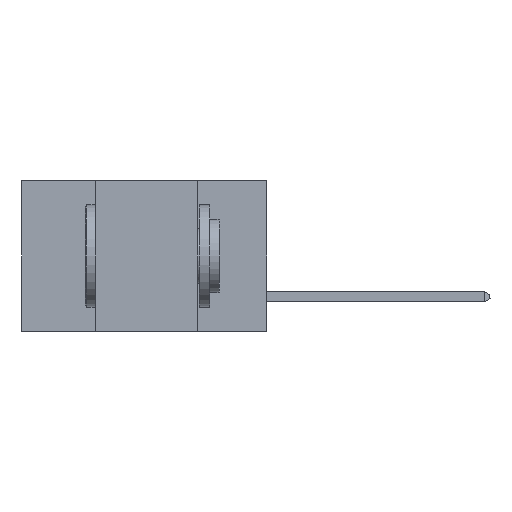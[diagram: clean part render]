
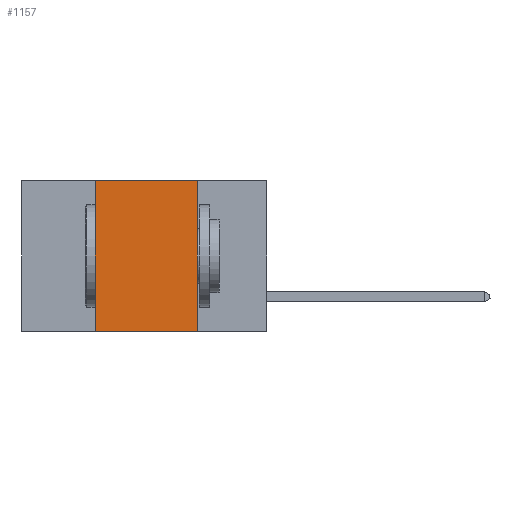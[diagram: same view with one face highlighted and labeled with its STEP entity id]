
A CAD part, left-side view. The second image highlights one B-rep face of the part: STEP entity #1157.
In plain terms, the highlighted planar face has unit normal (-1, 0, 0).
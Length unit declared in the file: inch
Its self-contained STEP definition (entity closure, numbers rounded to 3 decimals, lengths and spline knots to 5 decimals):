
#490 = ORIENTED_EDGE ( 'NONE', *, *, #20803, .F. ) ;
#624 = LINE ( 'NONE', #4602, #13449 ) ;
#963 = CARTESIAN_POINT ( 'NONE',  ( 0., 0.42, -0.37 ) ) ;
#1157 = ADVANCED_FACE ( 'NONE', ( #11332 ), #4888, .F. ) ;
#2945 = DIRECTION ( 'NONE',  ( 0., 0., 1. ) ) ;
#3739 = DIRECTION ( 'NONE',  ( 0., 0., -1. ) ) ;
#4158 = VERTEX_POINT ( 'NONE', #963 ) ;
#4268 = DIRECTION ( 'NONE',  ( 1., 0., 0. ) ) ;
#4602 = CARTESIAN_POINT ( 'NONE',  ( 0., 0.42, 0. ) ) ;
#4737 = CARTESIAN_POINT ( 'NONE',  ( 0., 0.6, 0. ) ) ;
#4888 = PLANE ( 'NONE',  #20525 ) ;
#5513 = VERTEX_POINT ( 'NONE', #19071 ) ;
#6127 = LINE ( 'NONE', #12574, #18599 ) ;
#7442 = EDGE_CURVE ( 'NONE', #8798, #15457, #12345, .T. ) ;
#8257 = DIRECTION ( 'NONE',  ( 0., -1., 0. ) ) ;
#8798 = VERTEX_POINT ( 'NONE', #10194 ) ;
#8953 = VECTOR ( 'NONE', #15605, 39.37008 ) ;
#10194 = CARTESIAN_POINT ( 'NONE',  ( 0., 0.17, 0. ) ) ;
#11332 = FACE_OUTER_BOUND ( 'NONE', #11573, .T. ) ;
#11573 = EDGE_LOOP ( 'NONE', ( #13331, #490, #14331, #18552 ) ) ;
#12345 = LINE ( 'NONE', #14002, #8953 ) ;
#12574 = CARTESIAN_POINT ( 'NONE',  ( 0., 0.6, 0. ) ) ;
#13331 = ORIENTED_EDGE ( 'NONE', *, *, #7442, .F. ) ;
#13449 = VECTOR ( 'NONE', #2945, 39.37008 ) ;
#14002 = CARTESIAN_POINT ( 'NONE',  ( 0., 0.17, 0. ) ) ;
#14241 = CARTESIAN_POINT ( 'NONE',  ( 0., 0.17, -0.37 ) ) ;
#14331 = ORIENTED_EDGE ( 'NONE', *, *, #19194, .F. ) ;
#15457 = VERTEX_POINT ( 'NONE', #14241 ) ;
#15605 = DIRECTION ( 'NONE',  ( 0., 0., -1. ) ) ;
#16250 = VECTOR ( 'NONE', #8257, 39.37008 ) ;
#17320 = DIRECTION ( 'NONE',  ( 0., -1., 0. ) ) ;
#18121 = EDGE_CURVE ( 'NONE', #4158, #15457, #20985, .T. ) ;
#18552 = ORIENTED_EDGE ( 'NONE', *, *, #18121, .T. ) ;
#18599 = VECTOR ( 'NONE', #17320, 39.37008 ) ;
#19071 = CARTESIAN_POINT ( 'NONE',  ( 0., 0.42, 0. ) ) ;
#19194 = EDGE_CURVE ( 'NONE', #4158, #5513, #624, .T. ) ;
#19566 = CARTESIAN_POINT ( 'NONE',  ( 0., 0.6, -0.37 ) ) ;
#20525 = AXIS2_PLACEMENT_3D ( 'NONE', #4737, #4268, #3739 ) ;
#20803 = EDGE_CURVE ( 'NONE', #5513, #8798, #6127, .T. ) ;
#20985 = LINE ( 'NONE', #19566, #16250 ) ;
